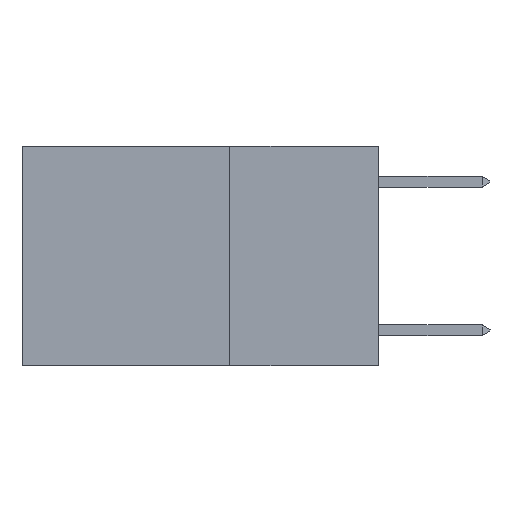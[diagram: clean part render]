
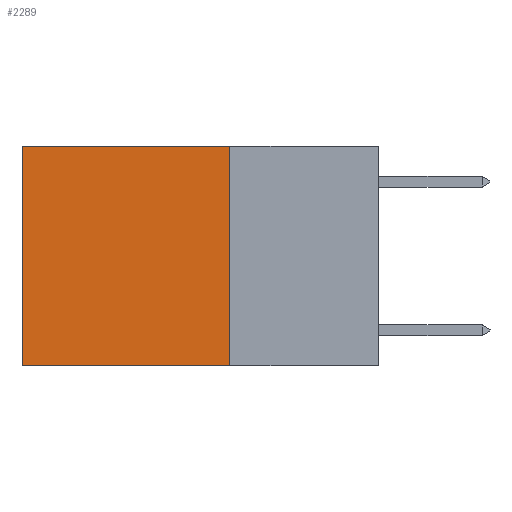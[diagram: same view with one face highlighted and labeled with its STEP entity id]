
A CAD part, left-side view. The second image highlights one B-rep face of the part: STEP entity #2289.
In plain terms, the highlighted planar face has unit normal (-1, 0, 0).
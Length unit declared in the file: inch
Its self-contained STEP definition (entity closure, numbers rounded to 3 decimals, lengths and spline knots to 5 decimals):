
#32 = DIRECTION ( 'NONE',  ( 0., 1., 0. ) ) ;
#40 = CARTESIAN_POINT ( 'NONE',  ( 0.2625, 0.25, 0. ) ) ;
#635 = LINE ( 'NONE', #17058, #16906 ) ;
#1879 = DIRECTION ( 'NONE',  ( 0., 0., -1. ) ) ;
#2289 = ADVANCED_FACE ( 'NONE', ( #15700 ), #2460, .F. ) ;
#2460 = PLANE ( 'NONE',  #18599 ) ;
#2829 = EDGE_LOOP ( 'NONE', ( #16672, #3787, #18719, #20306 ) ) ;
#3274 = CARTESIAN_POINT ( 'NONE',  ( 0.2625, 0.6, 0. ) ) ;
#3736 = DIRECTION ( 'NONE',  ( 0., 0., -1. ) ) ;
#3787 = ORIENTED_EDGE ( 'NONE', *, *, #6535, .F. ) ;
#6535 = EDGE_CURVE ( 'NONE', #9242, #15958, #22342, .T. ) ;
#7346 = VERTEX_POINT ( 'NONE', #25687 ) ;
#8613 = EDGE_CURVE ( 'NONE', #12079, #7346, #16903, .T. ) ;
#9166 = CARTESIAN_POINT ( 'NONE',  ( 0.2625, 0.25, -0.37 ) ) ;
#9242 = VERTEX_POINT ( 'NONE', #9166 ) ;
#11270 = EDGE_CURVE ( 'NONE', #12079, #9242, #635, .T. ) ;
#12079 = VERTEX_POINT ( 'NONE', #13014 ) ;
#12267 = CARTESIAN_POINT ( 'NONE',  ( 0.2625, 0.25, -0.37 ) ) ;
#13014 = CARTESIAN_POINT ( 'NONE',  ( 0.2625, 0.25, 0. ) ) ;
#13217 = DIRECTION ( 'NONE',  ( 0., 1., 0. ) ) ;
#14415 = LINE ( 'NONE', #3274, #23334 ) ;
#15078 = CARTESIAN_POINT ( 'NONE',  ( 0.2625, 0.25, 0. ) ) ;
#15341 = EDGE_CURVE ( 'NONE', #7346, #15958, #14415, .T. ) ;
#15700 = FACE_OUTER_BOUND ( 'NONE', #2829, .T. ) ;
#15958 = VERTEX_POINT ( 'NONE', #18483 ) ;
#16672 = ORIENTED_EDGE ( 'NONE', *, *, #15341, .T. ) ;
#16903 = LINE ( 'NONE', #15078, #18293 ) ;
#16906 = VECTOR ( 'NONE', #20864, 39.37008 ) ;
#17058 = CARTESIAN_POINT ( 'NONE',  ( 0.2625, 0.25, 0. ) ) ;
#18293 = VECTOR ( 'NONE', #13217, 39.37008 ) ;
#18483 = CARTESIAN_POINT ( 'NONE',  ( 0.2625, 0.6, -0.37 ) ) ;
#18599 = AXIS2_PLACEMENT_3D ( 'NONE', #40, #20616, #3736 ) ;
#18719 = ORIENTED_EDGE ( 'NONE', *, *, #11270, .F. ) ;
#20306 = ORIENTED_EDGE ( 'NONE', *, *, #8613, .T. ) ;
#20616 = DIRECTION ( 'NONE',  ( 1., 0., 0. ) ) ;
#20864 = DIRECTION ( 'NONE',  ( 0., 0., -1. ) ) ;
#22342 = LINE ( 'NONE', #12267, #23764 ) ;
#23334 = VECTOR ( 'NONE', #1879, 39.37008 ) ;
#23764 = VECTOR ( 'NONE', #32, 39.37008 ) ;
#25687 = CARTESIAN_POINT ( 'NONE',  ( 0.2625, 0.6, 0. ) ) ;
